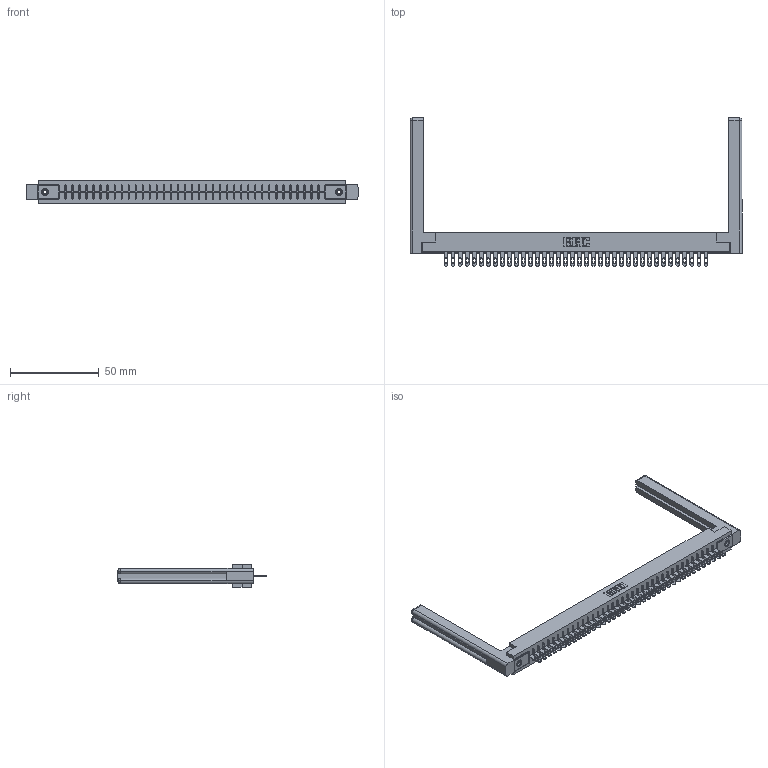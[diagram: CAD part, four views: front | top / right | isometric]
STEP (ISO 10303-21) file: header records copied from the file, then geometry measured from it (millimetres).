
FILE_DESCRIPTION (( 'STEP AP203' ), '1' );
FILE_NAME ('356-038-500-158.STEP', '2018-08-01T22:10:58', ( '' ), ( '' ), 'SwSTEP 2.0', 'SolidWorks 2016', '' );
FILE_SCHEMA (( 'CONFIG_CONTROL_DESIGN' ));
Length unit declared in the file: inch
Products named in the file (5): 306 Part_.156 Dia; 306-290-001_100; 345-250-001_345-250-001-102; 307-220-058; 356-038-500-158
Assembly tree (43 placements, depth 2):
  356-038-500-158
    306 Part_.156 Dia
    306-290-001_100  x38
    345-250-001_345-250-001-102  x2
    307-220-058  x2
Bounding box: 187.2 x 83.52 x 12.7 mm (x, y, z)
Volume: 27858.5 mm3; surface area: 27088.4 mm2
Topology: 43 solids, 43 shells, 3146 faces, 8840 edges, 5676 vertices
Faces by surface type: plane 2052, cylinder 918, sphere 152, cone 12, torus 12
Entity records: 38752 total; most frequent: CARTESIAN_POINT 6516, ORIENTED_EDGE 6402, DIRECTION 6381, EDGE_CURVE 3201, LINE 2495, VECTOR 2495, VERTEX_POINT 2024, AXIS2_PLACEMENT_3D 1943
